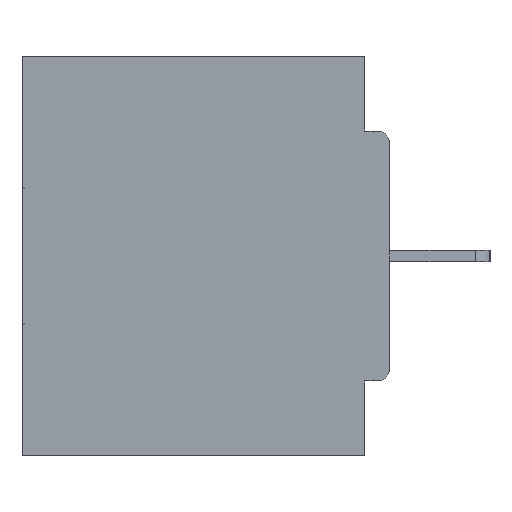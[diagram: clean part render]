
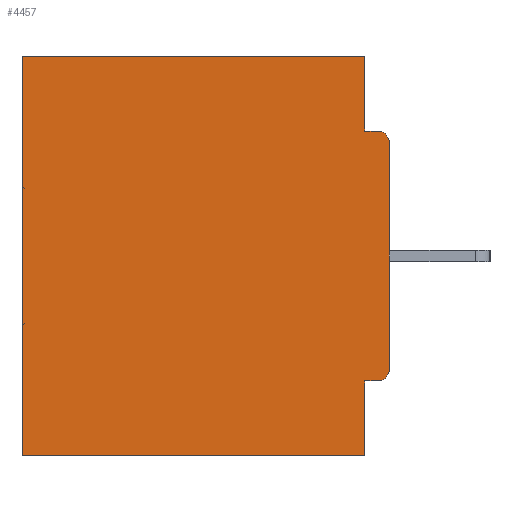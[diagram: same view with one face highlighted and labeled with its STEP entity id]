
A CAD part, left-side view. The second image highlights one B-rep face of the part: STEP entity #4457.
In plain terms, the highlighted planar face has unit normal (-1, 0, 0).
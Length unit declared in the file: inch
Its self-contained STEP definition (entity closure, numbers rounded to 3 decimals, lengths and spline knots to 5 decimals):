
#778 = ORIENTED_EDGE ( 'NONE', *, *, #32208, .T. ) ;
#874 = LINE ( 'NONE', #26229, #3091 ) ;
#1038 = LINE ( 'NONE', #14510, #16297 ) ;
#2258 = CARTESIAN_POINT ( 'NONE',  ( 0.298, 0.031, -0.5 ) ) ;
#2372 = DIRECTION ( 'NONE',  ( 0., 0., -1. ) ) ;
#2866 = EDGE_CURVE ( 'NONE', #29909, #3484, #6818, .T. ) ;
#3091 = VECTOR ( 'NONE', #17964, 39.37008 ) ;
#3132 = LINE ( 'NONE', #12112, #9555 ) ;
#3153 = ORIENTED_EDGE ( 'NONE', *, *, #18414, .F. ) ;
#3484 = VERTEX_POINT ( 'NONE', #8206 ) ;
#4100 = AXIS2_PLACEMENT_3D ( 'NONE', #16157, #32975, #12982 ) ;
#4457 = ADVANCED_FACE ( 'NONE', ( #5793 ), #30449, .F. ) ;
#4553 = CARTESIAN_POINT ( 'NONE',  ( 0.298, 0.46, 0. ) ) ;
#5130 = CARTESIAN_POINT ( 'NONE',  ( 0.298, 0.015, -0.3915 ) ) ;
#5201 = DIRECTION ( 'NONE',  ( 0., 0., -1. ) ) ;
#5497 = EDGE_CURVE ( 'NONE', #20187, #3484, #32682, .T. ) ;
#5619 = ORIENTED_EDGE ( 'NONE', *, *, #33088, .T. ) ;
#5650 = CARTESIAN_POINT ( 'NONE',  ( 0.298, 0.031, -0.5 ) ) ;
#5793 = FACE_OUTER_BOUND ( 'NONE', #7637, .T. ) ;
#6533 = AXIS2_PLACEMENT_3D ( 'NONE', #33955, #22399, #5201 ) ;
#6742 = AXIS2_PLACEMENT_3D ( 'NONE', #5130, #31276, #2372 ) ;
#6818 = LINE ( 'NONE', #10589, #9509 ) ;
#7637 = EDGE_LOOP ( 'NONE', ( #17025, #31793, #21401, #778, #36101, #26909, #13404, #33936, #5619, #3153 ) ) ;
#7982 = DIRECTION ( 'NONE',  ( 0., -1., 0. ) ) ;
#8206 = CARTESIAN_POINT ( 'NONE',  ( 0.298, 0.015, -0.0935 ) ) ;
#8533 = DIRECTION ( 'NONE',  ( 0., 0., -1. ) ) ;
#9509 = VECTOR ( 'NONE', #7982, 39.37008 ) ;
#9555 = VECTOR ( 'NONE', #17915, 39.37008 ) ;
#10192 = CARTESIAN_POINT ( 'NONE',  ( 0.298, 0.031, -0.0935 ) ) ;
#10589 = CARTESIAN_POINT ( 'NONE',  ( 0.298, 0., -0.0935 ) ) ;
#11874 = LINE ( 'NONE', #5650, #19034 ) ;
#12112 = CARTESIAN_POINT ( 'NONE',  ( 0.298, 0., -0.5 ) ) ;
#12896 = CIRCLE ( 'NONE', #6742, 0.015 ) ;
#12982 = DIRECTION ( 'NONE',  ( 0., 0., -1. ) ) ;
#13404 = ORIENTED_EDGE ( 'NONE', *, *, #20492, .F. ) ;
#13684 = EDGE_CURVE ( 'NONE', #29057, #16439, #3132, .T. ) ;
#14510 = CARTESIAN_POINT ( 'NONE',  ( 0.298, 0., -0.4065 ) ) ;
#15161 = CARTESIAN_POINT ( 'NONE',  ( 0.298, 0.031, -0.5 ) ) ;
#15756 = CARTESIAN_POINT ( 'NONE',  ( 0.298, 0.031, 0. ) ) ;
#15798 = LINE ( 'NONE', #34460, #22500 ) ;
#16157 = CARTESIAN_POINT ( 'NONE',  ( 0.298, 0., 0. ) ) ;
#16297 = VECTOR ( 'NONE', #20310, 39.37008 ) ;
#16439 = VERTEX_POINT ( 'NONE', #25997 ) ;
#17025 = ORIENTED_EDGE ( 'NONE', *, *, #5497, .T. ) ;
#17915 = DIRECTION ( 'NONE',  ( 0., 1., 0. ) ) ;
#17964 = DIRECTION ( 'NONE',  ( 0., 0., -1. ) ) ;
#18086 = VERTEX_POINT ( 'NONE', #4553 ) ;
#18414 = EDGE_CURVE ( 'NONE', #20187, #34798, #874, .T. ) ;
#19034 = VECTOR ( 'NONE', #8533, 39.37008 ) ;
#20187 = VERTEX_POINT ( 'NONE', #35955 ) ;
#20310 = DIRECTION ( 'NONE',  ( 0., 1., 0. ) ) ;
#20492 = EDGE_CURVE ( 'NONE', #32478, #29057, #36985, .T. ) ;
#20767 = EDGE_CURVE ( 'NONE', #24778, #32478, #1038, .T. ) ;
#21401 = ORIENTED_EDGE ( 'NONE', *, *, #30706, .F. ) ;
#22399 = DIRECTION ( 'NONE',  ( -1., 0., 0. ) ) ;
#22500 = VECTOR ( 'NONE', #34329, 39.37008 ) ;
#22976 = VERTEX_POINT ( 'NONE', #15756 ) ;
#24238 = CARTESIAN_POINT ( 'NONE',  ( 0.298, 0.031, -0.4065 ) ) ;
#24778 = VERTEX_POINT ( 'NONE', #31731 ) ;
#25220 = DIRECTION ( 'NONE',  ( 0., 0., -1. ) ) ;
#25234 = EDGE_CURVE ( 'NONE', #18086, #16439, #29436, .T. ) ;
#25459 = DIRECTION ( 'NONE',  ( 0., 0., -1. ) ) ;
#25997 = CARTESIAN_POINT ( 'NONE',  ( 0.298, 0.46, -0.5 ) ) ;
#26175 = CARTESIAN_POINT ( 'NONE',  ( 0.298, 0., -0.3915 ) ) ;
#26229 = CARTESIAN_POINT ( 'NONE',  ( 0.298, 0., 0. ) ) ;
#26909 = ORIENTED_EDGE ( 'NONE', *, *, #13684, .F. ) ;
#28200 = CARTESIAN_POINT ( 'NONE',  ( 0.298, 0.46, 0. ) ) ;
#29057 = VERTEX_POINT ( 'NONE', #15161 ) ;
#29436 = LINE ( 'NONE', #28200, #33048 ) ;
#29909 = VERTEX_POINT ( 'NONE', #10192 ) ;
#30449 = PLANE ( 'NONE',  #4100 ) ;
#30672 = VECTOR ( 'NONE', #25220, 39.37008 ) ;
#30706 = EDGE_CURVE ( 'NONE', #22976, #29909, #11874, .T. ) ;
#31276 = DIRECTION ( 'NONE',  ( -1., 0., 0. ) ) ;
#31731 = CARTESIAN_POINT ( 'NONE',  ( 0.298, 0.015, -0.4065 ) ) ;
#31793 = ORIENTED_EDGE ( 'NONE', *, *, #2866, .F. ) ;
#32208 = EDGE_CURVE ( 'NONE', #22976, #18086, #15798, .T. ) ;
#32478 = VERTEX_POINT ( 'NONE', #24238 ) ;
#32682 = CIRCLE ( 'NONE', #6533, 0.015 ) ;
#32975 = DIRECTION ( 'NONE',  ( 1., 0., 0. ) ) ;
#33048 = VECTOR ( 'NONE', #25459, 39.37008 ) ;
#33088 = EDGE_CURVE ( 'NONE', #24778, #34798, #12896, .T. ) ;
#33936 = ORIENTED_EDGE ( 'NONE', *, *, #20767, .F. ) ;
#33955 = CARTESIAN_POINT ( 'NONE',  ( 0.298, 0.015, -0.1085 ) ) ;
#34329 = DIRECTION ( 'NONE',  ( 0., 1., 0. ) ) ;
#34460 = CARTESIAN_POINT ( 'NONE',  ( 0.298, 0., 0. ) ) ;
#34798 = VERTEX_POINT ( 'NONE', #26175 ) ;
#35955 = CARTESIAN_POINT ( 'NONE',  ( 0.298, 0., -0.1085 ) ) ;
#36101 = ORIENTED_EDGE ( 'NONE', *, *, #25234, .T. ) ;
#36985 = LINE ( 'NONE', #2258, #30672 ) ;
